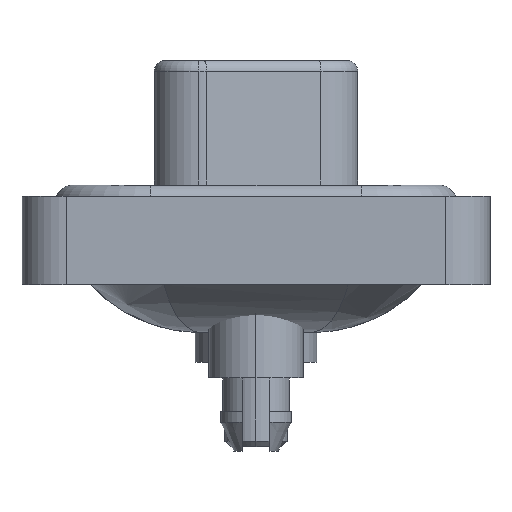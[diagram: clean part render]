
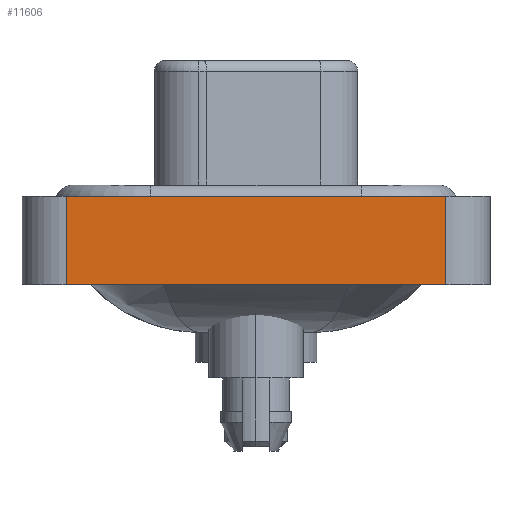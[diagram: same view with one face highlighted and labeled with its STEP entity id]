
A CAD part, left-side view. The second image highlights one B-rep face of the part: STEP entity #11606.
In plain terms, the highlighted planar face has unit normal (-1, 0, 0).
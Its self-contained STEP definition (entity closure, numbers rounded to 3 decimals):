
#8 = CARTESIAN_POINT ( 'NONE',  ( -7.3, -8.55, -3.6 ) ) ;
#738 = DIRECTION ( 'NONE',  ( 0., 0., 1. ) ) ;
#990 = CARTESIAN_POINT ( 'NONE',  ( -7.3, 8.55, -3.6 ) ) ;
#1679 = LINE ( 'NONE', #18229, #12588 ) ;
#2586 = VERTEX_POINT ( 'NONE', #13568 ) ;
#3008 = VERTEX_POINT ( 'NONE', #990 ) ;
#3897 = CARTESIAN_POINT ( 'NONE',  ( -7.3, 8.55, -3.6 ) ) ;
#4130 = EDGE_CURVE ( 'NONE', #3008, #7038, #9022, .T. ) ;
#5565 = EDGE_LOOP ( 'NONE', ( #16738, #7585, #12935, #9412 ) ) ;
#6379 = VERTEX_POINT ( 'NONE', #7044 ) ;
#6657 = FACE_OUTER_BOUND ( 'NONE', #5565, .T. ) ;
#7038 = VERTEX_POINT ( 'NONE', #20596 ) ;
#7044 = CARTESIAN_POINT ( 'NONE',  ( -7.3, -8.55, -3.6 ) ) ;
#7585 = ORIENTED_EDGE ( 'NONE', *, *, #10635, .F. ) ;
#8102 = CARTESIAN_POINT ( 'NONE',  ( -7.3, -8.55, -3.6 ) ) ;
#8117 = VECTOR ( 'NONE', #10058, 1000. ) ;
#8373 = VECTOR ( 'NONE', #16130, 1000. ) ;
#9022 = LINE ( 'NONE', #3897, #10645 ) ;
#9412 = ORIENTED_EDGE ( 'NONE', *, *, #19788, .T. ) ;
#9749 = LINE ( 'NONE', #8102, #8117 ) ;
#10058 = DIRECTION ( 'NONE',  ( 0., -1., 0. ) ) ;
#10635 = EDGE_CURVE ( 'NONE', #7038, #2586, #1679, .T. ) ;
#10645 = VECTOR ( 'NONE', #738, 1000. ) ;
#11606 = ADVANCED_FACE ( 'NONE', ( #6657 ), #18285, .T. ) ;
#12588 = VECTOR ( 'NONE', #14956, 1000. ) ;
#12935 = ORIENTED_EDGE ( 'NONE', *, *, #4130, .F. ) ;
#13568 = CARTESIAN_POINT ( 'NONE',  ( -7.3, -8.55, 0.4 ) ) ;
#13895 = EDGE_CURVE ( 'NONE', #6379, #2586, #20887, .T. ) ;
#14806 = DIRECTION ( 'NONE',  ( -1., 0., 0. ) ) ;
#14956 = DIRECTION ( 'NONE',  ( 0., -1., 0. ) ) ;
#15905 = CARTESIAN_POINT ( 'NONE',  ( -7.3, -8.55, -3.6 ) ) ;
#16130 = DIRECTION ( 'NONE',  ( 0., 0., 1. ) ) ;
#16738 = ORIENTED_EDGE ( 'NONE', *, *, #13895, .T. ) ;
#17103 = AXIS2_PLACEMENT_3D ( 'NONE', #8, #14806, #21438 ) ;
#18229 = CARTESIAN_POINT ( 'NONE',  ( -7.3, -8.55, 0.4 ) ) ;
#18285 = PLANE ( 'NONE',  #17103 ) ;
#19788 = EDGE_CURVE ( 'NONE', #3008, #6379, #9749, .T. ) ;
#20596 = CARTESIAN_POINT ( 'NONE',  ( -7.3, 8.55, 0.4 ) ) ;
#20887 = LINE ( 'NONE', #15905, #8373 ) ;
#21438 = DIRECTION ( 'NONE',  ( 0., 0., 1. ) ) ;
